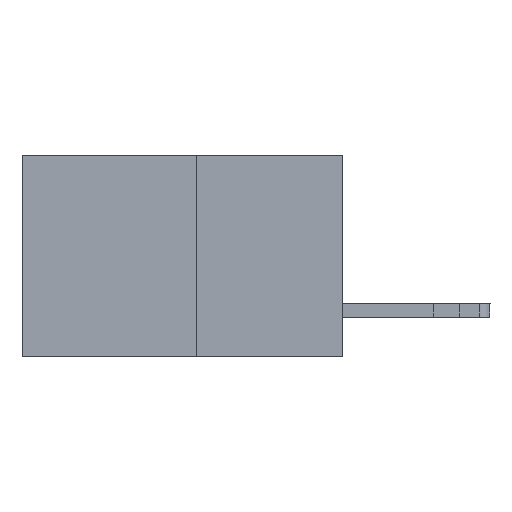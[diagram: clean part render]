
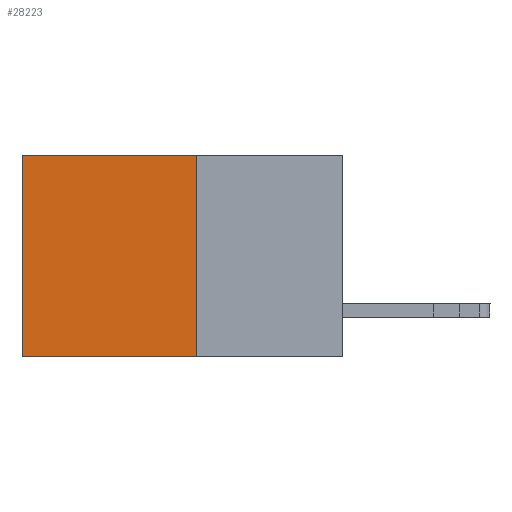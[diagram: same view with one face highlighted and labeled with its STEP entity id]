
A CAD part, left-side view. The second image highlights one B-rep face of the part: STEP entity #28223.
In plain terms, the highlighted planar face has unit normal (-1, 0, 0).
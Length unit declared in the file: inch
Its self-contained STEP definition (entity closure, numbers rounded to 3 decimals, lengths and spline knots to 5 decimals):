
#78 = ORIENTED_EDGE ( 'NONE', *, *, #13657, .F. ) ;
#538 = LINE ( 'NONE', #16858, #26826 ) ;
#4105 = CARTESIAN_POINT ( 'NONE',  ( 0.277, 0.59, 0. ) ) ;
#4432 = VERTEX_POINT ( 'NONE', #20872 ) ;
#4578 = DIRECTION ( 'NONE',  ( 0., 0., -1. ) ) ;
#5145 = DIRECTION ( 'NONE',  ( 0., 1., 0. ) ) ;
#5206 = CARTESIAN_POINT ( 'NONE',  ( 0.277, 0.59, -0.37 ) ) ;
#5256 = CARTESIAN_POINT ( 'NONE',  ( 0.277, 0.27, 0. ) ) ;
#6021 = EDGE_CURVE ( 'NONE', #8508, #6807, #538, .T. ) ;
#6791 = EDGE_CURVE ( 'NONE', #4432, #8508, #9238, .T. ) ;
#6807 = VERTEX_POINT ( 'NONE', #5206 ) ;
#7038 = CARTESIAN_POINT ( 'NONE',  ( 0.277, 0.27, -0.37 ) ) ;
#7168 = PLANE ( 'NONE',  #15265 ) ;
#8508 = VERTEX_POINT ( 'NONE', #4105 ) ;
#9238 = LINE ( 'NONE', #5256, #14896 ) ;
#9347 = LINE ( 'NONE', #7038, #26870 ) ;
#10805 = FACE_OUTER_BOUND ( 'NONE', #16941, .T. ) ;
#11124 = VERTEX_POINT ( 'NONE', #29688 ) ;
#12012 = CARTESIAN_POINT ( 'NONE',  ( 0.277, 0.27, -0.37 ) ) ;
#13657 = EDGE_CURVE ( 'NONE', #4432, #11124, #9347, .T. ) ;
#14423 = DIRECTION ( 'NONE',  ( 0., 0., -1. ) ) ;
#14872 = ORIENTED_EDGE ( 'NONE', *, *, #6021, .T. ) ;
#14896 = VECTOR ( 'NONE', #5145, 39.37008 ) ;
#14980 = CARTESIAN_POINT ( 'NONE',  ( 0.277, 0.27, -0.37 ) ) ;
#15265 = AXIS2_PLACEMENT_3D ( 'NONE', #12012, #28607, #14423 ) ;
#16766 = DIRECTION ( 'NONE',  ( 0., 0., -1. ) ) ;
#16858 = CARTESIAN_POINT ( 'NONE',  ( 0.277, 0.59, -0.37 ) ) ;
#16941 = EDGE_LOOP ( 'NONE', ( #14872, #25275, #78, #22193 ) ) ;
#20872 = CARTESIAN_POINT ( 'NONE',  ( 0.277, 0.27, 0. ) ) ;
#22193 = ORIENTED_EDGE ( 'NONE', *, *, #6791, .T. ) ;
#23352 = VECTOR ( 'NONE', #26816, 39.37008 ) ;
#25275 = ORIENTED_EDGE ( 'NONE', *, *, #30150, .F. ) ;
#26816 = DIRECTION ( 'NONE',  ( 0., 1., 0. ) ) ;
#26826 = VECTOR ( 'NONE', #16766, 39.37008 ) ;
#26870 = VECTOR ( 'NONE', #4578, 39.37008 ) ;
#28223 = ADVANCED_FACE ( 'NONE', ( #10805 ), #7168, .F. ) ;
#28607 = DIRECTION ( 'NONE',  ( 1., 0., 0. ) ) ;
#29688 = CARTESIAN_POINT ( 'NONE',  ( 0.277, 0.27, -0.37 ) ) ;
#30150 = EDGE_CURVE ( 'NONE', #11124, #6807, #30266, .T. ) ;
#30266 = LINE ( 'NONE', #14980, #23352 ) ;
